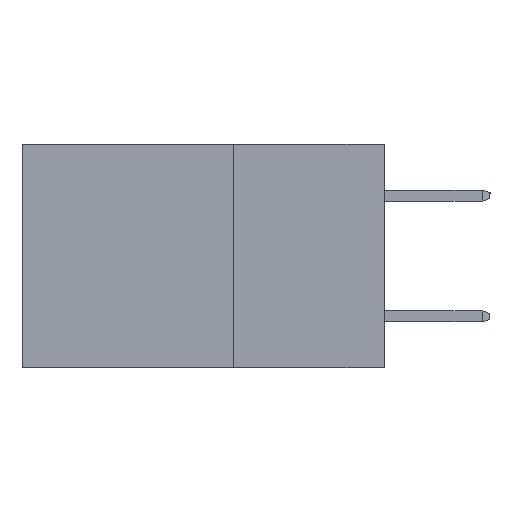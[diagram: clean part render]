
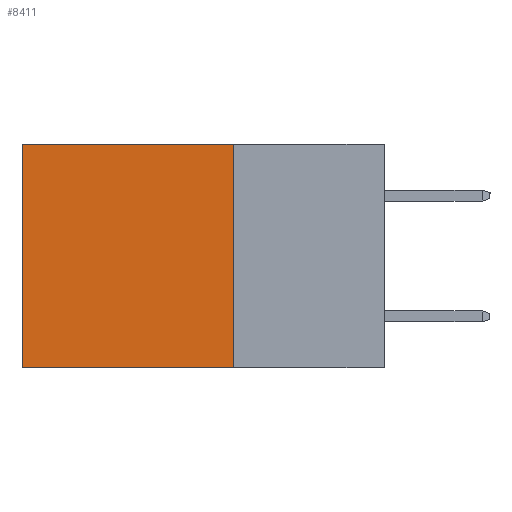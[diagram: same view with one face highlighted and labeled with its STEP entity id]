
A CAD part, left-side view. The second image highlights one B-rep face of the part: STEP entity #8411.
In plain terms, the highlighted planar face has unit normal (-1, 0, 0).
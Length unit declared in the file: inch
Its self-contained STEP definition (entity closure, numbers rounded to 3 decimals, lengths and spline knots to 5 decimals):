
#297 = EDGE_CURVE ( 'NONE', #7935, #6955, #10105, .T. ) ;
#501 = LINE ( 'NONE', #4866, #900 ) ;
#900 = VECTOR ( 'NONE', #9477, 39.37008 ) ;
#1047 = ORIENTED_EDGE ( 'NONE', *, *, #5248, .T. ) ;
#1774 = FACE_OUTER_BOUND ( 'NONE', #1790, .T. ) ;
#1790 = EDGE_LOOP ( 'NONE', ( #1047, #10385, #3420, #13152 ) ) ;
#2513 = AXIS2_PLACEMENT_3D ( 'NONE', #13497, #8651, #3053 ) ;
#2518 = DIRECTION ( 'NONE',  ( 0., 1., 0. ) ) ;
#3053 = DIRECTION ( 'NONE',  ( 0., 0., -1. ) ) ;
#3420 = ORIENTED_EDGE ( 'NONE', *, *, #297, .F. ) ;
#3795 = VECTOR ( 'NONE', #2518, 39.37008 ) ;
#4002 = VECTOR ( 'NONE', #11635, 39.37008 ) ;
#4866 = CARTESIAN_POINT ( 'NONE',  ( 0.2615, 0.6, -0.37 ) ) ;
#5095 = CARTESIAN_POINT ( 'NONE',  ( 0.2615, 0.6, 0. ) ) ;
#5248 = EDGE_CURVE ( 'NONE', #12590, #8187, #501, .T. ) ;
#5598 = EDGE_CURVE ( 'NONE', #6955, #8187, #7261, .T. ) ;
#5633 = CARTESIAN_POINT ( 'NONE',  ( 0.2615, 0.25, -0.37 ) ) ;
#5708 = CARTESIAN_POINT ( 'NONE',  ( 0.2615, 0.25, 0. ) ) ;
#6472 = DIRECTION ( 'NONE',  ( 0., 0., -1. ) ) ;
#6955 = VERTEX_POINT ( 'NONE', #14760 ) ;
#7261 = LINE ( 'NONE', #13181, #3795 ) ;
#7854 = CARTESIAN_POINT ( 'NONE',  ( 0.2615, 0.25, 0. ) ) ;
#7935 = VERTEX_POINT ( 'NONE', #5708 ) ;
#8134 = CARTESIAN_POINT ( 'NONE',  ( 0.2615, 0.6, -0.37 ) ) ;
#8187 = VERTEX_POINT ( 'NONE', #8134 ) ;
#8411 = ADVANCED_FACE ( 'NONE', ( #1774 ), #11278, .F. ) ;
#8651 = DIRECTION ( 'NONE',  ( 1., 0., 0. ) ) ;
#9477 = DIRECTION ( 'NONE',  ( 0., 0., -1. ) ) ;
#10105 = LINE ( 'NONE', #5633, #13547 ) ;
#10342 = EDGE_CURVE ( 'NONE', #7935, #12590, #10502, .T. ) ;
#10385 = ORIENTED_EDGE ( 'NONE', *, *, #5598, .F. ) ;
#10502 = LINE ( 'NONE', #7854, #4002 ) ;
#11278 = PLANE ( 'NONE',  #2513 ) ;
#11635 = DIRECTION ( 'NONE',  ( 0., 1., 0. ) ) ;
#12590 = VERTEX_POINT ( 'NONE', #5095 ) ;
#13152 = ORIENTED_EDGE ( 'NONE', *, *, #10342, .T. ) ;
#13181 = CARTESIAN_POINT ( 'NONE',  ( 0.2615, 0.25, -0.37 ) ) ;
#13497 = CARTESIAN_POINT ( 'NONE',  ( 0.2615, 0.25, -0.37 ) ) ;
#13547 = VECTOR ( 'NONE', #6472, 39.37008 ) ;
#14760 = CARTESIAN_POINT ( 'NONE',  ( 0.2615, 0.25, -0.37 ) ) ;
